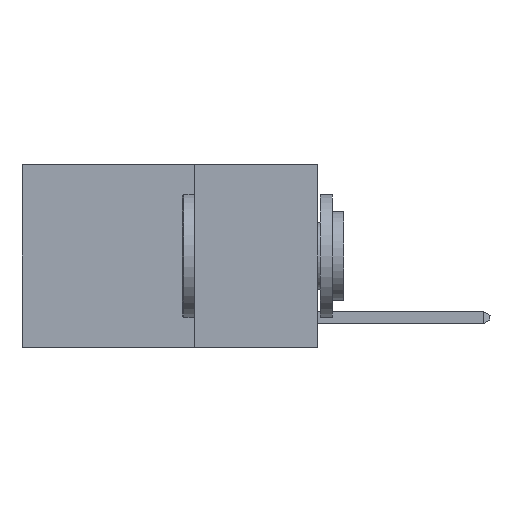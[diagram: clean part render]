
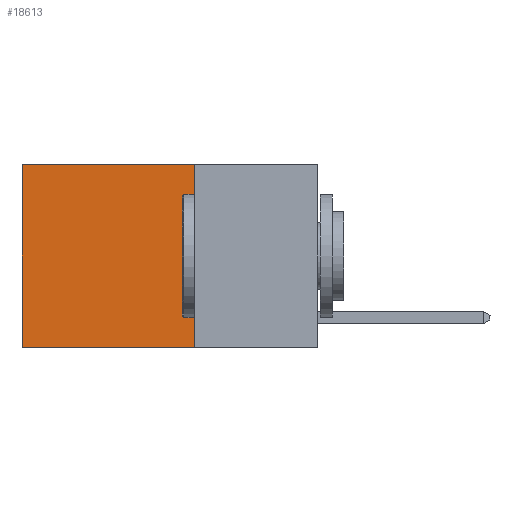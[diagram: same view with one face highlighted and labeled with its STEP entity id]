
A CAD part, left-side view. The second image highlights one B-rep face of the part: STEP entity #18613.
In plain terms, the highlighted planar face has unit normal (-1, 0, 0).
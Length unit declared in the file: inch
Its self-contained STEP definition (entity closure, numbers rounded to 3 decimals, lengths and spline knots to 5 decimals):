
#67 = DIRECTION ( 'NONE',  ( 0., 1., 0. ) ) ;
#377 = DIRECTION ( 'NONE',  ( 0., 1., 0. ) ) ;
#1647 = DIRECTION ( 'NONE',  ( 0., 0., -1. ) ) ;
#1742 = LINE ( 'NONE', #8191, #17193 ) ;
#2310 = EDGE_CURVE ( 'NONE', #13644, #20461, #1742, .T. ) ;
#3439 = ORIENTED_EDGE ( 'NONE', *, *, #16090, .T. ) ;
#3958 = VECTOR ( 'NONE', #1647, 39.37008 ) ;
#5129 = CARTESIAN_POINT ( 'NONE',  ( 0.2625, 0.25, -0.37 ) ) ;
#5253 = ORIENTED_EDGE ( 'NONE', *, *, #2310, .T. ) ;
#5350 = EDGE_CURVE ( 'NONE', #13644, #6987, #9562, .T. ) ;
#5423 = EDGE_LOOP ( 'NONE', ( #3439, #6784, #5545, #5253 ) ) ;
#5545 = ORIENTED_EDGE ( 'NONE', *, *, #5350, .F. ) ;
#5923 = CARTESIAN_POINT ( 'NONE',  ( 0.2625, 0.25, -0.37 ) ) ;
#6784 = ORIENTED_EDGE ( 'NONE', *, *, #9435, .F. ) ;
#6987 = VERTEX_POINT ( 'NONE', #5923 ) ;
#8191 = CARTESIAN_POINT ( 'NONE',  ( 0.2625, 0.25, 0. ) ) ;
#8793 = LINE ( 'NONE', #18583, #17362 ) ;
#9435 = EDGE_CURVE ( 'NONE', #6987, #14942, #14510, .T. ) ;
#9562 = LINE ( 'NONE', #15989, #3958 ) ;
#10563 = CARTESIAN_POINT ( 'NONE',  ( 0.2625, 0.6, -0.37 ) ) ;
#10933 = CARTESIAN_POINT ( 'NONE',  ( 0.2625, 0.25, 0. ) ) ;
#12203 = PLANE ( 'NONE',  #14223 ) ;
#12315 = DIRECTION ( 'NONE',  ( 0., 0., -1. ) ) ;
#13644 = VERTEX_POINT ( 'NONE', #10933 ) ;
#14014 = FACE_OUTER_BOUND ( 'NONE', #5423, .T. ) ;
#14223 = AXIS2_PLACEMENT_3D ( 'NONE', #15277, #20039, #12315 ) ;
#14510 = LINE ( 'NONE', #5129, #15515 ) ;
#14942 = VERTEX_POINT ( 'NONE', #10563 ) ;
#15277 = CARTESIAN_POINT ( 'NONE',  ( 0.2625, 0.25, 0. ) ) ;
#15515 = VECTOR ( 'NONE', #67, 39.37008 ) ;
#15989 = CARTESIAN_POINT ( 'NONE',  ( 0.2625, 0.25, 0. ) ) ;
#16090 = EDGE_CURVE ( 'NONE', #20461, #14942, #8793, .T. ) ;
#16948 = CARTESIAN_POINT ( 'NONE',  ( 0.2625, 0.6, 0. ) ) ;
#17193 = VECTOR ( 'NONE', #377, 39.37008 ) ;
#17362 = VECTOR ( 'NONE', #18277, 39.37008 ) ;
#18277 = DIRECTION ( 'NONE',  ( 0., 0., -1. ) ) ;
#18583 = CARTESIAN_POINT ( 'NONE',  ( 0.2625, 0.6, 0. ) ) ;
#18613 = ADVANCED_FACE ( 'NONE', ( #14014 ), #12203, .F. ) ;
#20039 = DIRECTION ( 'NONE',  ( 1., 0., 0. ) ) ;
#20461 = VERTEX_POINT ( 'NONE', #16948 ) ;
